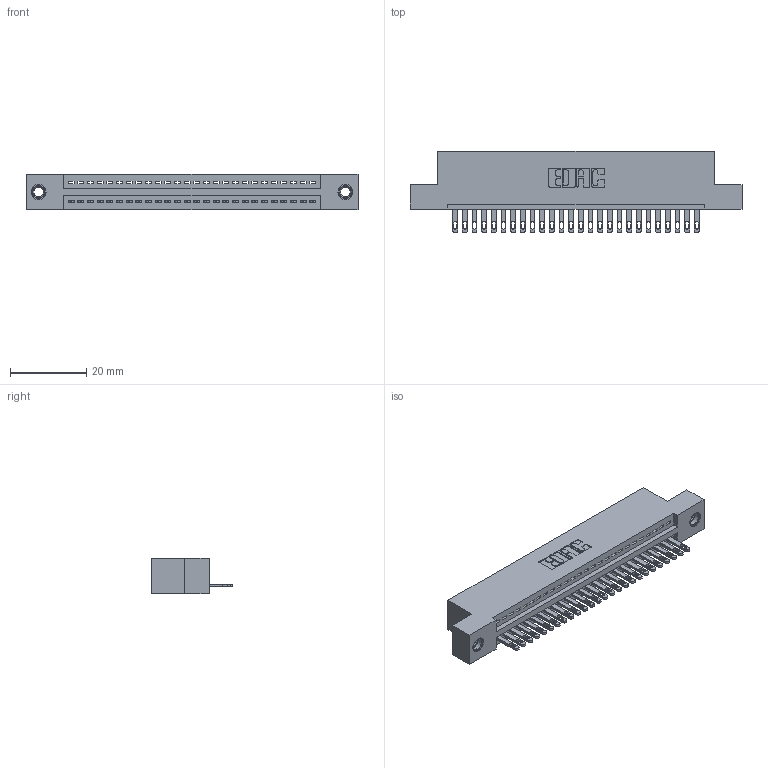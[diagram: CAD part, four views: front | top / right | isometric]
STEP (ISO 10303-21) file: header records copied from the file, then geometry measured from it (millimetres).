
FILE_DESCRIPTION (( 'STEP AP203' ), '1' );
FILE_NAME ('895-026-500-107.STEP', '2020-09-25T14:18:41', ( '' ), ( '' ), 'SwSTEP 2.0', 'SolidWorks 2020', '' );
FILE_SCHEMA (( 'CONFIG_CONTROL_DESIGN' ));
Length unit declared in the file: inch
Products named in the file (4): 345-292-001_345-293-100; 345-250-001_345-250-005-103; 895-026-500-107; 845 Part_Flush Mounting Lugs - 0.156 Dia-TI
Assembly tree (29 placements, depth 2):
  895-026-500-107
    845 Part_Flush Mounting Lugs - 0.156 Dia-TI
    345-292-001_345-293-100  x26
    345-250-001_345-250-005-103  x2
Bounding box: 87.25 x 21.51 x 9.4 mm (x, y, z)
Volume: 8158.5 mm3; surface area: 10715.4 mm2
Topology: 29 solids, 29 shells, 1590 faces, 4845 edges, 3222 vertices
Faces by surface type: plane 996, cylinder 578, cone 12, torus 4
Entity records: 22838 total; most frequent: CARTESIAN_POINT 3937, ORIENTED_EDGE 3890, DIRECTION 3491, EDGE_CURVE 1945, LINE 1685, VECTOR 1685, VERTEX_POINT 1292, AXIS2_PLACEMENT_3D 903
